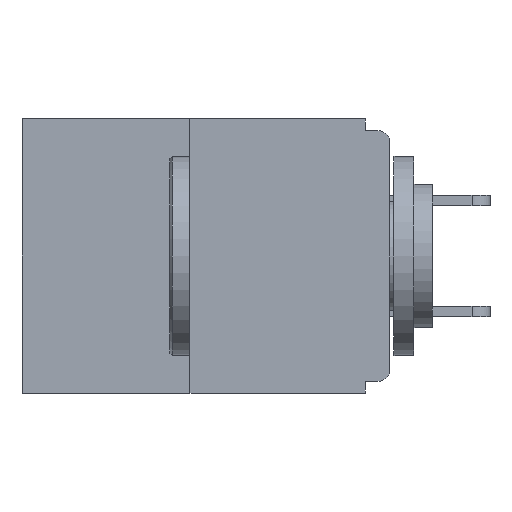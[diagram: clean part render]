
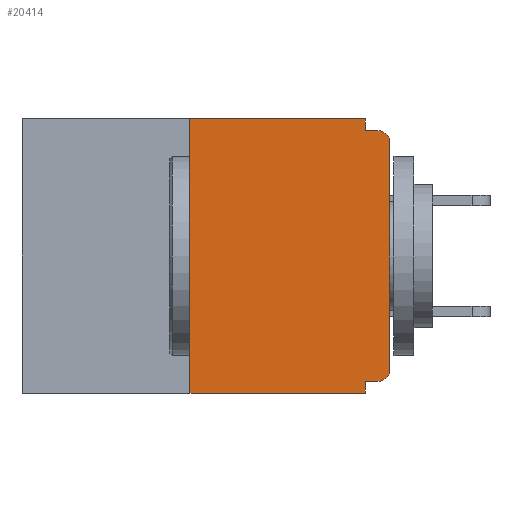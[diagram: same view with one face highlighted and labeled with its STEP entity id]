
A CAD part, left-side view. The second image highlights one B-rep face of the part: STEP entity #20414.
In plain terms, the highlighted planar face has unit normal (-1, 0, 0).
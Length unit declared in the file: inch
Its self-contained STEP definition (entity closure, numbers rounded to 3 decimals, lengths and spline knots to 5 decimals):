
#704 = ORIENTED_EDGE ( 'NONE', *, *, #13186, .F. ) ;
#832 = VERTEX_POINT ( 'NONE', #11303 ) ;
#941 = AXIS2_PLACEMENT_3D ( 'NONE', #11608, #15542, #7481 ) ;
#1111 = ORIENTED_EDGE ( 'NONE', *, *, #16580, .T. ) ;
#1129 = CARTESIAN_POINT ( 'NONE',  ( 0., 0.031, -0.015 ) ) ;
#1525 = CARTESIAN_POINT ( 'NONE',  ( 0., 0.015, -0.03 ) ) ;
#1581 = DIRECTION ( 'NONE',  ( 0., -1., 0. ) ) ;
#3168 = VERTEX_POINT ( 'NONE', #17738 ) ;
#3575 = CARTESIAN_POINT ( 'NONE',  ( 0., 0.031, 0. ) ) ;
#3803 = CARTESIAN_POINT ( 'NONE',  ( 0., 0.25, 0. ) ) ;
#4408 = ORIENTED_EDGE ( 'NONE', *, *, #25744, .T. ) ;
#4432 = ORIENTED_EDGE ( 'NONE', *, *, #13624, .F. ) ;
#6041 = DIRECTION ( 'NONE',  ( -1., 0., 0. ) ) ;
#6066 = ORIENTED_EDGE ( 'NONE', *, *, #23119, .T. ) ;
#6097 = EDGE_LOOP ( 'NONE', ( #27196, #704, #1111, #6417, #23028, #6066, #4408, #21330, #4432, #6655 ) ) ;
#6136 = AXIS2_PLACEMENT_3D ( 'NONE', #1525, #6041, #16206 ) ;
#6417 = ORIENTED_EDGE ( 'NONE', *, *, #13429, .F. ) ;
#6655 = ORIENTED_EDGE ( 'NONE', *, *, #10280, .F. ) ;
#7030 = VERTEX_POINT ( 'NONE', #12352 ) ;
#7068 = DIRECTION ( 'NONE',  ( -1., 0., 0. ) ) ;
#7106 = VERTEX_POINT ( 'NONE', #18883 ) ;
#7224 = PLANE ( 'NONE',  #941 ) ;
#7336 = AXIS2_PLACEMENT_3D ( 'NONE', #11439, #7068, #21730 ) ;
#7481 = DIRECTION ( 'NONE',  ( 0., 0., -1. ) ) ;
#7793 = DIRECTION ( 'NONE',  ( 0., 1., 0. ) ) ;
#8011 = CARTESIAN_POINT ( 'NONE',  ( 0., 0.031, -0.343 ) ) ;
#8296 = VECTOR ( 'NONE', #12360, 39.37008 ) ;
#8974 = EDGE_CURVE ( 'NONE', #832, #10149, #26985, .T. ) ;
#9140 = VERTEX_POINT ( 'NONE', #16676 ) ;
#9532 = VECTOR ( 'NONE', #22858, 39.37008 ) ;
#10149 = VERTEX_POINT ( 'NONE', #16624 ) ;
#10203 = DIRECTION ( 'NONE',  ( 0., 0., 1. ) ) ;
#10214 = VECTOR ( 'NONE', #20563, 39.37008 ) ;
#10279 = VERTEX_POINT ( 'NONE', #26357 ) ;
#10280 = EDGE_CURVE ( 'NONE', #10149, #15615, #18694, .T. ) ;
#10802 = VECTOR ( 'NONE', #22186, 39.37008 ) ;
#11303 = CARTESIAN_POINT ( 'NONE',  ( 0., 0.25, 0. ) ) ;
#11439 = CARTESIAN_POINT ( 'NONE',  ( 0., 0.015, -0.313 ) ) ;
#11608 = CARTESIAN_POINT ( 'NONE',  ( 0., 0.46, 0. ) ) ;
#12134 = CARTESIAN_POINT ( 'NONE',  ( 0., 0., -0.015 ) ) ;
#12352 = CARTESIAN_POINT ( 'NONE',  ( 0., 0.25, -0.343 ) ) ;
#12360 = DIRECTION ( 'NONE',  ( 0., 0., -1. ) ) ;
#12976 = EDGE_CURVE ( 'NONE', #9140, #13579, #25106, .T. ) ;
#13186 = EDGE_CURVE ( 'NONE', #7030, #832, #22767, .T. ) ;
#13220 = LINE ( 'NONE', #15969, #23723 ) ;
#13429 = EDGE_CURVE ( 'NONE', #3168, #13906, #13874, .T. ) ;
#13579 = VERTEX_POINT ( 'NONE', #27142 ) ;
#13583 = VECTOR ( 'NONE', #10203, 39.37008 ) ;
#13624 = EDGE_CURVE ( 'NONE', #15615, #13579, #17179, .T. ) ;
#13697 = DIRECTION ( 'NONE',  ( 0., 0., 1. ) ) ;
#13874 = LINE ( 'NONE', #26691, #8296 ) ;
#13906 = VERTEX_POINT ( 'NONE', #8011 ) ;
#14713 = CIRCLE ( 'NONE', #7336, 0.015 ) ;
#15542 = DIRECTION ( 'NONE',  ( 1., 0., 0. ) ) ;
#15615 = VERTEX_POINT ( 'NONE', #1129 ) ;
#15969 = CARTESIAN_POINT ( 'NONE',  ( 0., 0., -0.328 ) ) ;
#16183 = VECTOR ( 'NONE', #1581, 39.37008 ) ;
#16206 = DIRECTION ( 'NONE',  ( 0., 0., -1. ) ) ;
#16434 = EDGE_CURVE ( 'NONE', #7106, #3168, #13220, .T. ) ;
#16462 = LINE ( 'NONE', #22955, #9532 ) ;
#16580 = EDGE_CURVE ( 'NONE', #7030, #13906, #16462, .T. ) ;
#16624 = CARTESIAN_POINT ( 'NONE',  ( 0., 0.031, 0. ) ) ;
#16676 = CARTESIAN_POINT ( 'NONE',  ( 0., 0., -0.03 ) ) ;
#17179 = LINE ( 'NONE', #12134, #16183 ) ;
#17651 = CARTESIAN_POINT ( 'NONE',  ( 0., 0., 0. ) ) ;
#17738 = CARTESIAN_POINT ( 'NONE',  ( 0., 0.031, -0.328 ) ) ;
#18694 = LINE ( 'NONE', #3575, #10802 ) ;
#18883 = CARTESIAN_POINT ( 'NONE',  ( 0., 0.015, -0.328 ) ) ;
#19254 = VECTOR ( 'NONE', #13697, 39.37008 ) ;
#20414 = ADVANCED_FACE ( 'NONE', ( #22367 ), #7224, .F. ) ;
#20563 = DIRECTION ( 'NONE',  ( 0., -1., 0. ) ) ;
#21330 = ORIENTED_EDGE ( 'NONE', *, *, #12976, .T. ) ;
#21730 = DIRECTION ( 'NONE',  ( 0., 0., -1. ) ) ;
#22186 = DIRECTION ( 'NONE',  ( 0., 0., -1. ) ) ;
#22367 = FACE_OUTER_BOUND ( 'NONE', #6097, .T. ) ;
#22642 = CARTESIAN_POINT ( 'NONE',  ( 0., 0.46, 0. ) ) ;
#22767 = LINE ( 'NONE', #3803, #13583 ) ;
#22858 = DIRECTION ( 'NONE',  ( 0., -1., 0. ) ) ;
#22955 = CARTESIAN_POINT ( 'NONE',  ( 0., 0.46, -0.343 ) ) ;
#23028 = ORIENTED_EDGE ( 'NONE', *, *, #16434, .F. ) ;
#23119 = EDGE_CURVE ( 'NONE', #7106, #10279, #14713, .T. ) ;
#23179 = LINE ( 'NONE', #17651, #19254 ) ;
#23723 = VECTOR ( 'NONE', #7793, 39.37008 ) ;
#25106 = CIRCLE ( 'NONE', #6136, 0.015 ) ;
#25744 = EDGE_CURVE ( 'NONE', #10279, #9140, #23179, .T. ) ;
#26357 = CARTESIAN_POINT ( 'NONE',  ( 0., 0., -0.313 ) ) ;
#26691 = CARTESIAN_POINT ( 'NONE',  ( 0., 0.031, -0.343 ) ) ;
#26985 = LINE ( 'NONE', #22642, #10214 ) ;
#27142 = CARTESIAN_POINT ( 'NONE',  ( 0., 0.015, -0.015 ) ) ;
#27196 = ORIENTED_EDGE ( 'NONE', *, *, #8974, .F. ) ;
